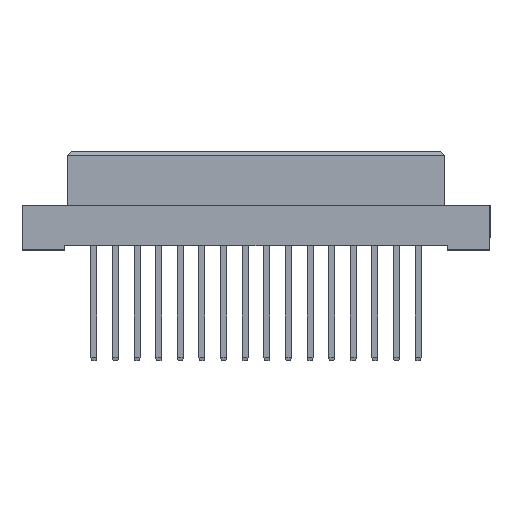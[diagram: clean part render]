
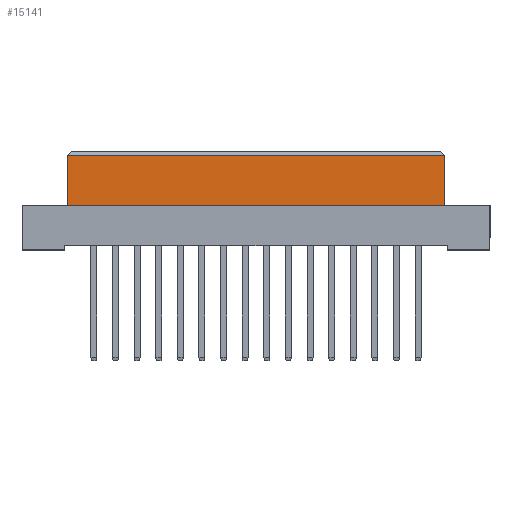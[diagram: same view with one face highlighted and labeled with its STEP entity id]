
A CAD part, top view. The second image highlights one B-rep face of the part: STEP entity #15141.
In plain terms, the highlighted planar face has unit normal (0, 0, 1).
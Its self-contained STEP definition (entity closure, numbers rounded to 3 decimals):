
#391 = PLANE ( 'NONE',  #18026 ) ;
#806 = CARTESIAN_POINT ( 'NONE',  ( 22.2, -6.4, 4.25 ) ) ;
#1504 = CARTESIAN_POINT ( 'NONE',  ( 22.2, -6.4, 4.25 ) ) ;
#1801 = CARTESIAN_POINT ( 'NONE',  ( -22.2, -6.4, 4.25 ) ) ;
#3041 = CARTESIAN_POINT ( 'NONE',  ( -22.2, -6.4, 4.25 ) ) ;
#4398 = CARTESIAN_POINT ( 'NONE',  ( 22.2, -0.5, 4.25 ) ) ;
#4745 = VERTEX_POINT ( 'NONE', #4398 ) ;
#5259 = VERTEX_POINT ( 'NONE', #13788 ) ;
#5761 = VERTEX_POINT ( 'NONE', #1801 ) ;
#6551 = CARTESIAN_POINT ( 'NONE',  ( 22.2, -6.4, 4.25 ) ) ;
#7010 = FACE_OUTER_BOUND ( 'NONE', #16819, .T. ) ;
#8196 = EDGE_CURVE ( 'NONE', #5259, #4745, #16172, .T. ) ;
#9736 = VECTOR ( 'NONE', #19640, 1000. ) ;
#10009 = DIRECTION ( 'NONE',  ( -1., 0., 0. ) ) ;
#11199 = VECTOR ( 'NONE', #11479, 1000. ) ;
#11479 = DIRECTION ( 'NONE',  ( 1., 0., 0. ) ) ;
#12809 = CARTESIAN_POINT ( 'NONE',  ( -22.2, -0.5, 4.25 ) ) ;
#12875 = ORIENTED_EDGE ( 'NONE', *, *, #14439, .F. ) ;
#13544 = DIRECTION ( 'NONE',  ( 0., 0., 1. ) ) ;
#13589 = ORIENTED_EDGE ( 'NONE', *, *, #8196, .T. ) ;
#13788 = CARTESIAN_POINT ( 'NONE',  ( 22.2, -6.4, 4.25 ) ) ;
#14439 = EDGE_CURVE ( 'NONE', #5761, #21173, #16507, .T. ) ;
#14608 = VECTOR ( 'NONE', #10009, 1000. ) ;
#15141 = ADVANCED_FACE ( 'NONE', ( #7010 ), #391, .T. ) ;
#16172 = LINE ( 'NONE', #1504, #21234 ) ;
#16490 = LINE ( 'NONE', #12809, #14608 ) ;
#16507 = LINE ( 'NONE', #3041, #9736 ) ;
#16819 = EDGE_LOOP ( 'NONE', ( #13589, #17243, #12875, #21064 ) ) ;
#17243 = ORIENTED_EDGE ( 'NONE', *, *, #17562, .T. ) ;
#17562 = EDGE_CURVE ( 'NONE', #4745, #21173, #16490, .T. ) ;
#17979 = EDGE_CURVE ( 'NONE', #5761, #5259, #19682, .T. ) ;
#18026 = AXIS2_PLACEMENT_3D ( 'NONE', #806, #13544, #20152 ) ;
#19640 = DIRECTION ( 'NONE',  ( 0., 1., 0. ) ) ;
#19682 = LINE ( 'NONE', #6551, #11199 ) ;
#19836 = DIRECTION ( 'NONE',  ( 0., 1., 0. ) ) ;
#20152 = DIRECTION ( 'NONE',  ( 1., 0., 0. ) ) ;
#20861 = CARTESIAN_POINT ( 'NONE',  ( -22.2, -0.5, 4.25 ) ) ;
#21064 = ORIENTED_EDGE ( 'NONE', *, *, #17979, .T. ) ;
#21173 = VERTEX_POINT ( 'NONE', #20861 ) ;
#21234 = VECTOR ( 'NONE', #19836, 1000. ) ;
